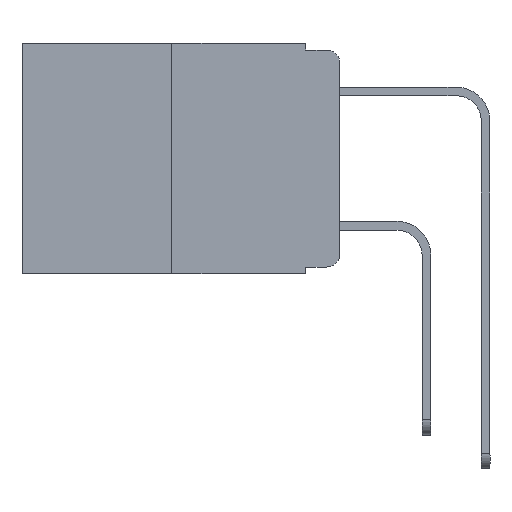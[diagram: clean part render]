
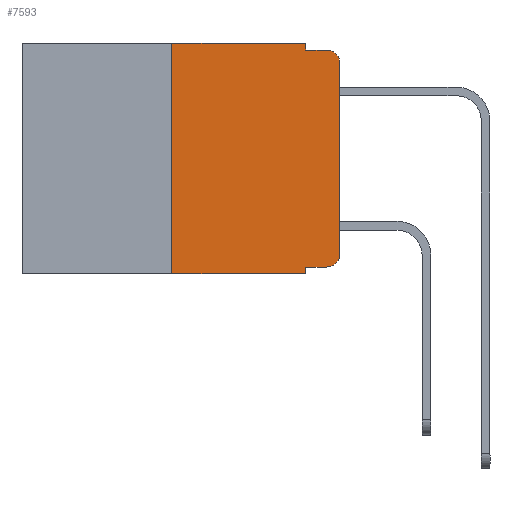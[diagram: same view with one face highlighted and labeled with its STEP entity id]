
A CAD part, left-side view. The second image highlights one B-rep face of the part: STEP entity #7593.
In plain terms, the highlighted planar face has unit normal (-1, 0, 0).
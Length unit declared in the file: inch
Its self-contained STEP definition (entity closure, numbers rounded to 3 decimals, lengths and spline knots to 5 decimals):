
#147 = DIRECTION ( 'NONE',  ( 0., 0., 1. ) ) ;
#236 = EDGE_CURVE ( 'NONE', #3895, #8707, #8088, .T. ) ;
#530 = VERTEX_POINT ( 'NONE', #14987 ) ;
#632 = CARTESIAN_POINT ( 'NONE',  ( 0., 0.02, -0.333 ) ) ;
#1004 = CARTESIAN_POINT ( 'NONE',  ( 0., 0.051, -0.343 ) ) ;
#1038 = AXIS2_PLACEMENT_3D ( 'NONE', #3080, #15509, #10360 ) ;
#1324 = LINE ( 'NONE', #14785, #6169 ) ;
#1549 = CARTESIAN_POINT ( 'NONE',  ( 0., 0.25, -0.343 ) ) ;
#1609 = CARTESIAN_POINT ( 'NONE',  ( 0., 0.02, -0.01 ) ) ;
#1769 = ORIENTED_EDGE ( 'NONE', *, *, #236, .F. ) ;
#1845 = VERTEX_POINT ( 'NONE', #632 ) ;
#2084 = VECTOR ( 'NONE', #7817, 39.37008 ) ;
#2101 = DIRECTION ( 'NONE',  ( 0., 0., -1. ) ) ;
#2167 = DIRECTION ( 'NONE',  ( 0., 0., -1. ) ) ;
#2180 = EDGE_CURVE ( 'NONE', #8817, #8707, #13844, .T. ) ;
#3080 = CARTESIAN_POINT ( 'NONE',  ( 0., 0.02, -0.313 ) ) ;
#3222 = VECTOR ( 'NONE', #8958, 39.37008 ) ;
#3280 = EDGE_CURVE ( 'NONE', #12104, #3308, #8795, .T. ) ;
#3308 = VERTEX_POINT ( 'NONE', #13953 ) ;
#3830 = VECTOR ( 'NONE', #147, 39.37008 ) ;
#3895 = VERTEX_POINT ( 'NONE', #11727 ) ;
#4298 = CARTESIAN_POINT ( 'NONE',  ( 0., 0.473, -0.343 ) ) ;
#4885 = CARTESIAN_POINT ( 'NONE',  ( 0., 0.051, -0.333 ) ) ;
#5363 = DIRECTION ( 'NONE',  ( 0., -1., 0. ) ) ;
#5694 = DIRECTION ( 'NONE',  ( 0., 0., -1. ) ) ;
#5813 = ORIENTED_EDGE ( 'NONE', *, *, #2180, .T. ) ;
#6169 = VECTOR ( 'NONE', #9861, 39.37008 ) ;
#6318 = CARTESIAN_POINT ( 'NONE',  ( 0., 0.25, 0. ) ) ;
#7059 = EDGE_CURVE ( 'NONE', #1845, #530, #14614, .T. ) ;
#7194 = CARTESIAN_POINT ( 'NONE',  ( 0., 0.051, 0. ) ) ;
#7401 = ORIENTED_EDGE ( 'NONE', *, *, #7059, .T. ) ;
#7593 = ADVANCED_FACE ( 'NONE', ( #13807 ), #7937, .F. ) ;
#7601 = LINE ( 'NONE', #8878, #3222 ) ;
#7746 = ORIENTED_EDGE ( 'NONE', *, *, #3280, .F. ) ;
#7817 = DIRECTION ( 'NONE',  ( 0., -1., 0. ) ) ;
#7937 = PLANE ( 'NONE',  #9820 ) ;
#7977 = ORIENTED_EDGE ( 'NONE', *, *, #8104, .F. ) ;
#8088 = LINE ( 'NONE', #7194, #9168 ) ;
#8104 = EDGE_CURVE ( 'NONE', #12793, #8109, #7601, .T. ) ;
#8109 = VERTEX_POINT ( 'NONE', #1609 ) ;
#8201 = VECTOR ( 'NONE', #2167, 39.37008 ) ;
#8261 = VECTOR ( 'NONE', #5363, 39.37008 ) ;
#8707 = VERTEX_POINT ( 'NONE', #1004 ) ;
#8795 = LINE ( 'NONE', #11454, #8261 ) ;
#8804 = EDGE_CURVE ( 'NONE', #530, #15266, #1324, .T. ) ;
#8817 = VERTEX_POINT ( 'NONE', #1549 ) ;
#8878 = CARTESIAN_POINT ( 'NONE',  ( 0., 0.051, -0.01 ) ) ;
#8958 = DIRECTION ( 'NONE',  ( 0., -1., 0. ) ) ;
#9168 = VECTOR ( 'NONE', #5694, 39.37008 ) ;
#9666 = LINE ( 'NONE', #4885, #10225 ) ;
#9668 = ORIENTED_EDGE ( 'NONE', *, *, #8804, .T. ) ;
#9820 = AXIS2_PLACEMENT_3D ( 'NONE', #12525, #11480, #12700 ) ;
#9861 = DIRECTION ( 'NONE',  ( 0., 0., 1. ) ) ;
#10225 = VECTOR ( 'NONE', #14752, 39.37008 ) ;
#10360 = DIRECTION ( 'NONE',  ( 0., 0., -1. ) ) ;
#10650 = LINE ( 'NONE', #11700, #8201 ) ;
#10745 = CIRCLE ( 'NONE', #14620, 0.02 ) ;
#11074 = EDGE_CURVE ( 'NONE', #3895, #1845, #9666, .T. ) ;
#11080 = ORIENTED_EDGE ( 'NONE', *, *, #11074, .T. ) ;
#11115 = EDGE_CURVE ( 'NONE', #8817, #12104, #14595, .T. ) ;
#11454 = CARTESIAN_POINT ( 'NONE',  ( 0., 0.473, 0. ) ) ;
#11480 = DIRECTION ( 'NONE',  ( 1., 0., 0. ) ) ;
#11562 = CARTESIAN_POINT ( 'NONE',  ( 0., 0.25, 0. ) ) ;
#11700 = CARTESIAN_POINT ( 'NONE',  ( 0., 0.051, 0. ) ) ;
#11727 = CARTESIAN_POINT ( 'NONE',  ( 0., 0.051, -0.333 ) ) ;
#12104 = VERTEX_POINT ( 'NONE', #11562 ) ;
#12115 = ORIENTED_EDGE ( 'NONE', *, *, #12206, .T. ) ;
#12206 = EDGE_CURVE ( 'NONE', #15266, #8109, #10745, .T. ) ;
#12525 = CARTESIAN_POINT ( 'NONE',  ( 0., 0.473, 0. ) ) ;
#12555 = CARTESIAN_POINT ( 'NONE',  ( 0., 0.051, -0.01 ) ) ;
#12700 = DIRECTION ( 'NONE',  ( 0., 0., -1. ) ) ;
#12773 = CARTESIAN_POINT ( 'NONE',  ( 0., 0.02, -0.03 ) ) ;
#12793 = VERTEX_POINT ( 'NONE', #12555 ) ;
#13531 = ORIENTED_EDGE ( 'NONE', *, *, #14012, .F. ) ;
#13807 = FACE_OUTER_BOUND ( 'NONE', #14278, .T. ) ;
#13844 = LINE ( 'NONE', #4298, #2084 ) ;
#13953 = CARTESIAN_POINT ( 'NONE',  ( 0., 0.051, 0. ) ) ;
#14012 = EDGE_CURVE ( 'NONE', #3308, #12793, #10650, .T. ) ;
#14278 = EDGE_LOOP ( 'NONE', ( #9668, #12115, #7977, #13531, #7746, #14839, #5813, #1769, #11080, #7401 ) ) ;
#14595 = LINE ( 'NONE', #6318, #3830 ) ;
#14599 = CARTESIAN_POINT ( 'NONE',  ( 0., 0., -0.03 ) ) ;
#14614 = CIRCLE ( 'NONE', #1038, 0.02 ) ;
#14620 = AXIS2_PLACEMENT_3D ( 'NONE', #12773, #14942, #2101 ) ;
#14752 = DIRECTION ( 'NONE',  ( 0., -1., 0. ) ) ;
#14785 = CARTESIAN_POINT ( 'NONE',  ( 0., 0., 0. ) ) ;
#14839 = ORIENTED_EDGE ( 'NONE', *, *, #11115, .F. ) ;
#14942 = DIRECTION ( 'NONE',  ( -1., 0., 0. ) ) ;
#14987 = CARTESIAN_POINT ( 'NONE',  ( 0., 0., -0.313 ) ) ;
#15266 = VERTEX_POINT ( 'NONE', #14599 ) ;
#15509 = DIRECTION ( 'NONE',  ( -1., 0., 0. ) ) ;
